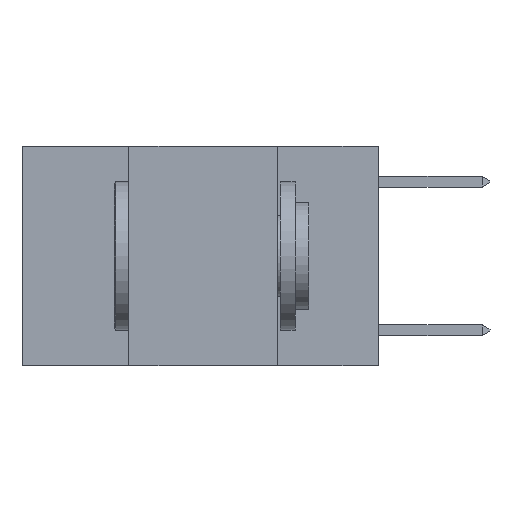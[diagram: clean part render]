
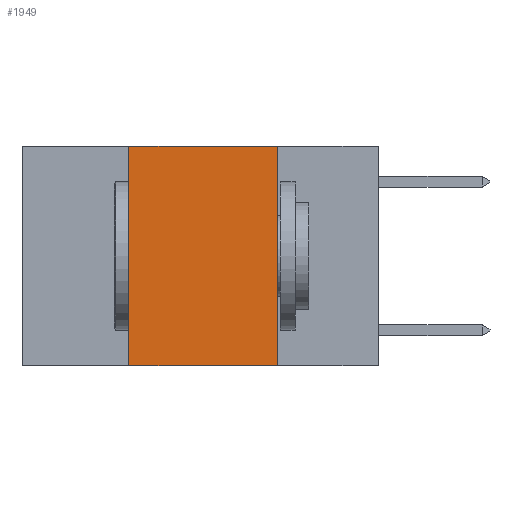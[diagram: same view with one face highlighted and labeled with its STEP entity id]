
A CAD part, left-side view. The second image highlights one B-rep face of the part: STEP entity #1949.
In plain terms, the highlighted planar face has unit normal (-1, 0, 0).
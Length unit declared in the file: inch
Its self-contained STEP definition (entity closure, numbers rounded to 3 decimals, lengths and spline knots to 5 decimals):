
#182 = EDGE_LOOP ( 'NONE', ( #902, #9870, #1090, #5567 ) ) ;
#845 = EDGE_CURVE ( 'NONE', #8238, #12361, #12741, .T. ) ;
#902 = ORIENTED_EDGE ( 'NONE', *, *, #7846, .F. ) ;
#1090 = ORIENTED_EDGE ( 'NONE', *, *, #845, .F. ) ;
#1403 = AXIS2_PLACEMENT_3D ( 'NONE', #7017, #4851, #4808 ) ;
#1682 = VECTOR ( 'NONE', #8144, 39.37008 ) ;
#1949 = ADVANCED_FACE ( 'NONE', ( #10826 ), #5328, .F. ) ;
#3172 = CARTESIAN_POINT ( 'NONE',  ( 0., 0.6, 0. ) ) ;
#3402 = LINE ( 'NONE', #3172, #6144 ) ;
#3938 = VERTEX_POINT ( 'NONE', #3948 ) ;
#3948 = CARTESIAN_POINT ( 'NONE',  ( 0., 0.17, -0.37 ) ) ;
#3963 = EDGE_CURVE ( 'NONE', #12361, #11445, #3402, .T. ) ;
#4581 = CARTESIAN_POINT ( 'NONE',  ( 0., 0.42, 0. ) ) ;
#4597 = VECTOR ( 'NONE', #5454, 39.37008 ) ;
#4754 = LINE ( 'NONE', #8228, #1682 ) ;
#4808 = DIRECTION ( 'NONE',  ( 0., 0., -1. ) ) ;
#4851 = DIRECTION ( 'NONE',  ( 1., 0., 0. ) ) ;
#5328 = PLANE ( 'NONE',  #1403 ) ;
#5454 = DIRECTION ( 'NONE',  ( 0., 0., 1. ) ) ;
#5567 = ORIENTED_EDGE ( 'NONE', *, *, #7946, .T. ) ;
#5717 = LINE ( 'NONE', #8816, #10845 ) ;
#6144 = VECTOR ( 'NONE', #11462, 39.37008 ) ;
#6265 = CARTESIAN_POINT ( 'NONE',  ( 0., 0.42, -0.37 ) ) ;
#7017 = CARTESIAN_POINT ( 'NONE',  ( 0., 0.6, 0. ) ) ;
#7846 = EDGE_CURVE ( 'NONE', #11445, #3938, #5717, .T. ) ;
#7946 = EDGE_CURVE ( 'NONE', #8238, #3938, #4754, .T. ) ;
#8144 = DIRECTION ( 'NONE',  ( 0., -1., 0. ) ) ;
#8228 = CARTESIAN_POINT ( 'NONE',  ( 0., 0.6, -0.37 ) ) ;
#8238 = VERTEX_POINT ( 'NONE', #6265 ) ;
#8816 = CARTESIAN_POINT ( 'NONE',  ( 0., 0.17, 0. ) ) ;
#8830 = DIRECTION ( 'NONE',  ( 0., 0., -1. ) ) ;
#9694 = CARTESIAN_POINT ( 'NONE',  ( 0., 0.42, 0. ) ) ;
#9870 = ORIENTED_EDGE ( 'NONE', *, *, #3963, .F. ) ;
#10274 = CARTESIAN_POINT ( 'NONE',  ( 0., 0.17, 0. ) ) ;
#10826 = FACE_OUTER_BOUND ( 'NONE', #182, .T. ) ;
#10845 = VECTOR ( 'NONE', #8830, 39.37008 ) ;
#11445 = VERTEX_POINT ( 'NONE', #10274 ) ;
#11462 = DIRECTION ( 'NONE',  ( 0., -1., 0. ) ) ;
#12361 = VERTEX_POINT ( 'NONE', #9694 ) ;
#12741 = LINE ( 'NONE', #4581, #4597 ) ;
